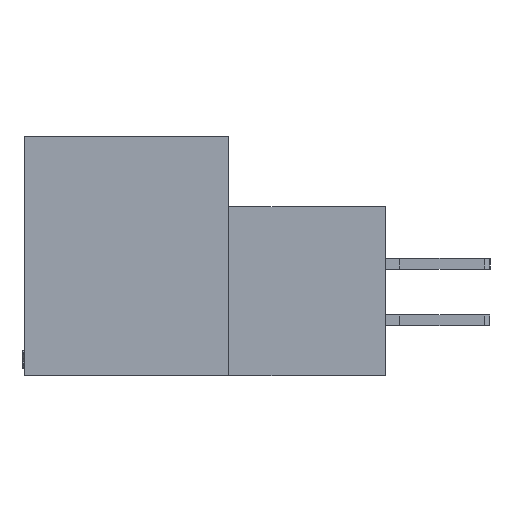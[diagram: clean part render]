
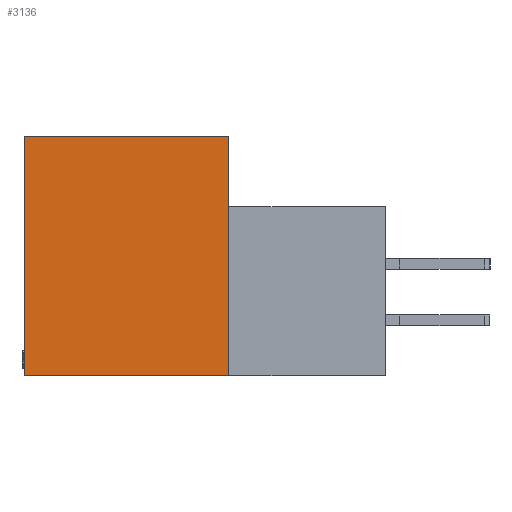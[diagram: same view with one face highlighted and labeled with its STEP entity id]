
A CAD part, left-side view. The second image highlights one B-rep face of the part: STEP entity #3136.
In plain terms, the highlighted planar face has unit normal (-1, 0, 0).
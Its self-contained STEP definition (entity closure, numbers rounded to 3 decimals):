
#2010 = CARTESIAN_POINT ( 'NONE',  ( 0., 11.506, -13.487 ) ) ;
#2836 = VERTEX_POINT ( 'NONE', #31026 ) ;
#3136 = ADVANCED_FACE ( 'NONE', ( #6882 ), #10942, .F. ) ;
#4825 = LINE ( 'NONE', #15365, #18693 ) ;
#6882 = FACE_OUTER_BOUND ( 'NONE', #13672, .T. ) ;
#7874 = CARTESIAN_POINT ( 'NONE',  ( 0., 11.506, 0. ) ) ;
#7892 = DIRECTION ( 'NONE',  ( 1., 0., 0. ) ) ;
#10409 = ORIENTED_EDGE ( 'NONE', *, *, #26843, .F. ) ;
#10567 = CARTESIAN_POINT ( 'NONE',  ( 0., 0., 0. ) ) ;
#10684 = DIRECTION ( 'NONE',  ( 0., 0., -1. ) ) ;
#10752 = LINE ( 'NONE', #7874, #24661 ) ;
#10840 = ORIENTED_EDGE ( 'NONE', *, *, #26362, .F. ) ;
#10942 = PLANE ( 'NONE',  #34418 ) ;
#12491 = VERTEX_POINT ( 'NONE', #2010 ) ;
#12566 = CARTESIAN_POINT ( 'NONE',  ( 0., 0., -13.487 ) ) ;
#12752 = LINE ( 'NONE', #10567, #16524 ) ;
#13672 = EDGE_LOOP ( 'NONE', ( #10409, #15721, #10840, #29359 ) ) ;
#14579 = VERTEX_POINT ( 'NONE', #23750 ) ;
#14888 = CARTESIAN_POINT ( 'NONE',  ( 0., 11.506, -13.487 ) ) ;
#15365 = CARTESIAN_POINT ( 'NONE',  ( 0., -8.814, -13.487 ) ) ;
#15721 = ORIENTED_EDGE ( 'NONE', *, *, #28294, .F. ) ;
#16524 = VECTOR ( 'NONE', #10684, 1000. ) ;
#17469 = DIRECTION ( 'NONE',  ( 0., 0., 1. ) ) ;
#18693 = VECTOR ( 'NONE', #20769, 1000. ) ;
#20143 = LINE ( 'NONE', #14888, #28952 ) ;
#20769 = DIRECTION ( 'NONE',  ( 0., 1., 0. ) ) ;
#21043 = DIRECTION ( 'NONE',  ( 0., -1., 0. ) ) ;
#22232 = VERTEX_POINT ( 'NONE', #12566 ) ;
#23750 = CARTESIAN_POINT ( 'NONE',  ( 0., 0., 0. ) ) ;
#23994 = CARTESIAN_POINT ( 'NONE',  ( 0., 0., 0. ) ) ;
#24661 = VECTOR ( 'NONE', #21043, 1000. ) ;
#26362 = EDGE_CURVE ( 'NONE', #2836, #14579, #10752, .T. ) ;
#26843 = EDGE_CURVE ( 'NONE', #22232, #12491, #4825, .T. ) ;
#28294 = EDGE_CURVE ( 'NONE', #14579, #22232, #12752, .T. ) ;
#28952 = VECTOR ( 'NONE', #17469, 1000. ) ;
#29359 = ORIENTED_EDGE ( 'NONE', *, *, #34487, .F. ) ;
#29835 = DIRECTION ( 'NONE',  ( 0., 0., -1. ) ) ;
#31026 = CARTESIAN_POINT ( 'NONE',  ( 0., 11.506, 0. ) ) ;
#34418 = AXIS2_PLACEMENT_3D ( 'NONE', #23994, #7892, #29835 ) ;
#34487 = EDGE_CURVE ( 'NONE', #12491, #2836, #20143, .T. ) ;
